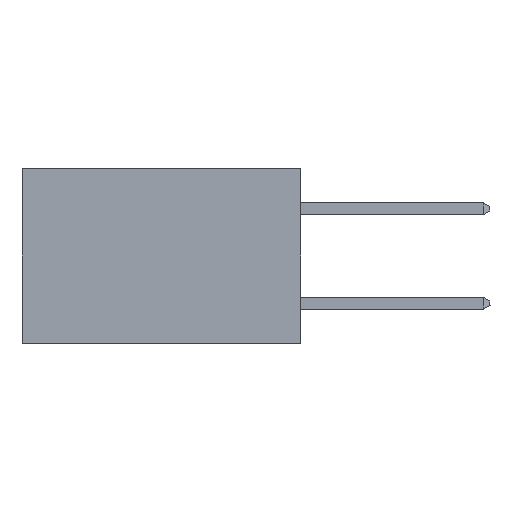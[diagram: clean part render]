
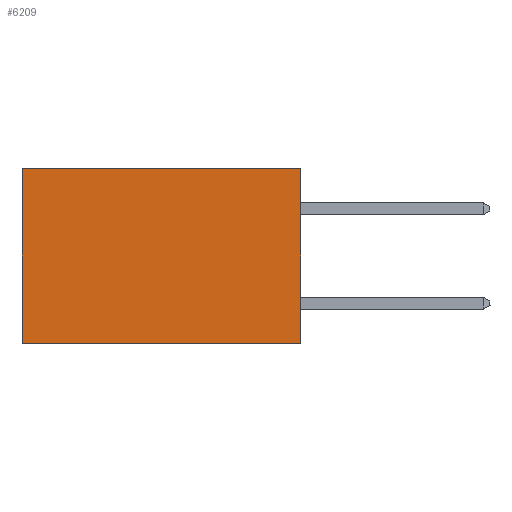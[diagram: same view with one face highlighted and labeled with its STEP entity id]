
A CAD part, left-side view. The second image highlights one B-rep face of the part: STEP entity #6209.
In plain terms, the highlighted planar face has unit normal (-1, 0, 0).
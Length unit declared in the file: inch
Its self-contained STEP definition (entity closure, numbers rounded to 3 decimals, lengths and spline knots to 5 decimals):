
#1406 = FACE_OUTER_BOUND ( 'NONE', #6042, .T. ) ;
#1628 = EDGE_CURVE ( 'NONE', #12678, #12300, #12289, .T. ) ;
#1788 = CARTESIAN_POINT ( 'NONE',  ( 0.277, 0.59, 0. ) ) ;
#3302 = DIRECTION ( 'NONE',  ( 0., 0., -1. ) ) ;
#3431 = DIRECTION ( 'NONE',  ( 1., 0., 0. ) ) ;
#3441 = DIRECTION ( 'NONE',  ( 0., 1., 0. ) ) ;
#3512 = CARTESIAN_POINT ( 'NONE',  ( 0.277, 0., 0. ) ) ;
#3526 = CARTESIAN_POINT ( 'NONE',  ( 0.277, 0., -0.37 ) ) ;
#3767 = LINE ( 'NONE', #11760, #7407 ) ;
#3833 = CARTESIAN_POINT ( 'NONE',  ( 0.277, 0., -0.37 ) ) ;
#5081 = PLANE ( 'NONE',  #9376 ) ;
#5492 = VERTEX_POINT ( 'NONE', #1788 ) ;
#6042 = EDGE_LOOP ( 'NONE', ( #10559, #18333, #11192, #12497 ) ) ;
#6209 = ADVANCED_FACE ( 'NONE', ( #1406 ), #5081, .F. ) ;
#7200 = EDGE_CURVE ( 'NONE', #12300, #12314, #16371, .T. ) ;
#7407 = VECTOR ( 'NONE', #10245, 39.37008 ) ;
#7647 = VECTOR ( 'NONE', #10232, 39.37008 ) ;
#9376 = AXIS2_PLACEMENT_3D ( 'NONE', #3526, #3431, #3302 ) ;
#9959 = CARTESIAN_POINT ( 'NONE',  ( 0.277, 0., -0.37 ) ) ;
#10232 = DIRECTION ( 'NONE',  ( 0., 0., -1. ) ) ;
#10245 = DIRECTION ( 'NONE',  ( 0., 1., 0. ) ) ;
#10559 = ORIENTED_EDGE ( 'NONE', *, *, #11586, .T. ) ;
#11146 = LINE ( 'NONE', #16656, #14755 ) ;
#11192 = ORIENTED_EDGE ( 'NONE', *, *, #1628, .F. ) ;
#11586 = EDGE_CURVE ( 'NONE', #5492, #12314, #11146, .T. ) ;
#11760 = CARTESIAN_POINT ( 'NONE',  ( 0.277, 0., 0. ) ) ;
#12289 = LINE ( 'NONE', #9959, #7647 ) ;
#12300 = VERTEX_POINT ( 'NONE', #16525 ) ;
#12314 = VERTEX_POINT ( 'NONE', #13503 ) ;
#12367 = VECTOR ( 'NONE', #3441, 39.37008 ) ;
#12497 = ORIENTED_EDGE ( 'NONE', *, *, #16726, .T. ) ;
#12678 = VERTEX_POINT ( 'NONE', #3512 ) ;
#13503 = CARTESIAN_POINT ( 'NONE',  ( 0.277, 0.59, -0.37 ) ) ;
#14755 = VECTOR ( 'NONE', #18172, 39.37008 ) ;
#16371 = LINE ( 'NONE', #3833, #12367 ) ;
#16525 = CARTESIAN_POINT ( 'NONE',  ( 0.277, 0., -0.37 ) ) ;
#16656 = CARTESIAN_POINT ( 'NONE',  ( 0.277, 0.59, -0.37 ) ) ;
#16726 = EDGE_CURVE ( 'NONE', #12678, #5492, #3767, .T. ) ;
#18172 = DIRECTION ( 'NONE',  ( 0., 0., -1. ) ) ;
#18333 = ORIENTED_EDGE ( 'NONE', *, *, #7200, .F. ) ;
